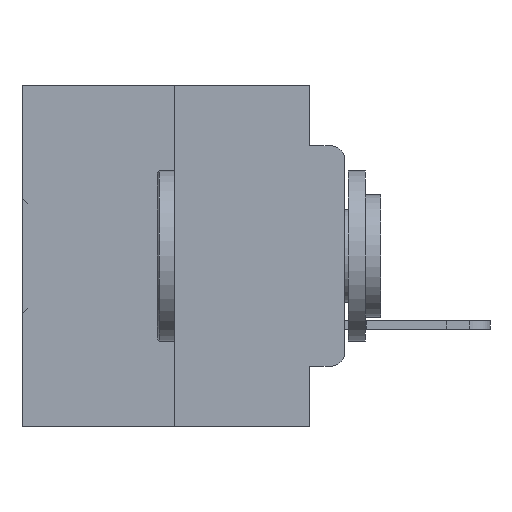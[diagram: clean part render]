
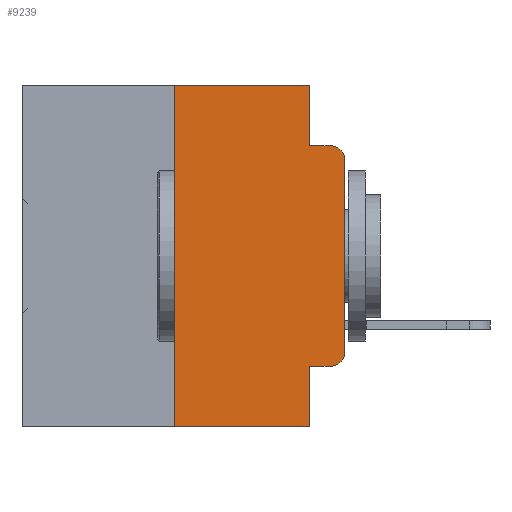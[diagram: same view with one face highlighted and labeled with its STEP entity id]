
A CAD part, left-side view. The second image highlights one B-rep face of the part: STEP entity #9239.
In plain terms, the highlighted planar face has unit normal (-1, 0, 0).
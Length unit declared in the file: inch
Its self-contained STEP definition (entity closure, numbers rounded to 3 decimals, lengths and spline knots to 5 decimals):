
#179 = VECTOR ( 'NONE', #11334, 39.37008 ) ;
#973 = FACE_OUTER_BOUND ( 'NONE', #3663, .T. ) ;
#1327 = CARTESIAN_POINT ( 'NONE',  ( 0., 0.051, -0.0885 ) ) ;
#1749 = CARTESIAN_POINT ( 'NONE',  ( 0., 0.473, 0. ) ) ;
#1759 = DIRECTION ( 'NONE',  ( 0., -1., 0. ) ) ;
#1784 = ORIENTED_EDGE ( 'NONE', *, *, #26303, .T. ) ;
#2339 = DIRECTION ( 'NONE',  ( 0., -1., 0. ) ) ;
#2803 = LINE ( 'NONE', #24411, #24666 ) ;
#3485 = CARTESIAN_POINT ( 'NONE',  ( 0., 0.473, -0.5 ) ) ;
#3663 = EDGE_LOOP ( 'NONE', ( #1784, #11729, #7660, #13972, #16989, #17748, #12508, #15870, #22640, #26390 ) ) ;
#3747 = VERTEX_POINT ( 'NONE', #17767 ) ;
#4022 = VERTEX_POINT ( 'NONE', #1327 ) ;
#4201 = VECTOR ( 'NONE', #25936, 39.37008 ) ;
#5179 = LINE ( 'NONE', #28516, #4201 ) ;
#5334 = CARTESIAN_POINT ( 'NONE',  ( 0., 0.051, -0.0885 ) ) ;
#5476 = VERTEX_POINT ( 'NONE', #19893 ) ;
#5604 = EDGE_CURVE ( 'NONE', #11550, #19818, #31973, .T. ) ;
#5982 = CARTESIAN_POINT ( 'NONE',  ( 0., 0.051, 0. ) ) ;
#6362 = LINE ( 'NONE', #28811, #13258 ) ;
#6499 = DIRECTION ( 'NONE',  ( 0., 0., -1. ) ) ;
#7012 = VERTEX_POINT ( 'NONE', #10464 ) ;
#7660 = ORIENTED_EDGE ( 'NONE', *, *, #20836, .F. ) ;
#8556 = PLANE ( 'NONE',  #15994 ) ;
#8940 = DIRECTION ( 'NONE',  ( 0., 0., 1. ) ) ;
#9149 = CARTESIAN_POINT ( 'NONE',  ( 0., 0.25, 0. ) ) ;
#9239 = ADVANCED_FACE ( 'NONE', ( #973 ), #8556, .F. ) ;
#10116 = EDGE_CURVE ( 'NONE', #14273, #35083, #30186, .T. ) ;
#10464 = CARTESIAN_POINT ( 'NONE',  ( 0., 0.02, -0.0885 ) ) ;
#11184 = LINE ( 'NONE', #5982, #18620 ) ;
#11334 = DIRECTION ( 'NONE',  ( 0., -1., 0. ) ) ;
#11550 = VERTEX_POINT ( 'NONE', #31933 ) ;
#11585 = EDGE_CURVE ( 'NONE', #20948, #11550, #6362, .T. ) ;
#11639 = CARTESIAN_POINT ( 'NONE',  ( 0., 0.25, -0.5 ) ) ;
#11729 = ORIENTED_EDGE ( 'NONE', *, *, #22694, .T. ) ;
#12382 = AXIS2_PLACEMENT_3D ( 'NONE', #14731, #14684, #14679 ) ;
#12508 = ORIENTED_EDGE ( 'NONE', *, *, #10116, .T. ) ;
#12522 = DIRECTION ( 'NONE',  ( 0., 0., -1. ) ) ;
#13258 = VECTOR ( 'NONE', #28668, 39.37008 ) ;
#13535 = EDGE_CURVE ( 'NONE', #20948, #35083, #2803, .T. ) ;
#13877 = DIRECTION ( 'NONE',  ( -1., 0., 0. ) ) ;
#13972 = ORIENTED_EDGE ( 'NONE', *, *, #19061, .F. ) ;
#14273 = VERTEX_POINT ( 'NONE', #11639 ) ;
#14632 = CARTESIAN_POINT ( 'NONE',  ( 0., 0., -0.3915 ) ) ;
#14679 = DIRECTION ( 'NONE',  ( 0., 0., -1. ) ) ;
#14684 = DIRECTION ( 'NONE',  ( -1., 0., 0. ) ) ;
#14731 = CARTESIAN_POINT ( 'NONE',  ( 0., 0.02, -0.3915 ) ) ;
#15371 = EDGE_CURVE ( 'NONE', #14273, #24079, #25806, .T. ) ;
#15619 = EDGE_CURVE ( 'NONE', #24079, #5476, #16378, .T. ) ;
#15870 = ORIENTED_EDGE ( 'NONE', *, *, #13535, .F. ) ;
#15994 = AXIS2_PLACEMENT_3D ( 'NONE', #35100, #34679, #12522 ) ;
#16378 = LINE ( 'NONE', #1749, #29738 ) ;
#16989 = ORIENTED_EDGE ( 'NONE', *, *, #15619, .F. ) ;
#17237 = AXIS2_PLACEMENT_3D ( 'NONE', #29869, #13877, #32298 ) ;
#17571 = CARTESIAN_POINT ( 'NONE',  ( 0., 0.051, -0.4115 ) ) ;
#17748 = ORIENTED_EDGE ( 'NONE', *, *, #15371, .F. ) ;
#17767 = CARTESIAN_POINT ( 'NONE',  ( 0., 0., -0.1085 ) ) ;
#18567 = VECTOR ( 'NONE', #8940, 39.37008 ) ;
#18620 = VECTOR ( 'NONE', #6499, 39.37008 ) ;
#19061 = EDGE_CURVE ( 'NONE', #5476, #4022, #11184, .T. ) ;
#19818 = VERTEX_POINT ( 'NONE', #14632 ) ;
#19893 = CARTESIAN_POINT ( 'NONE',  ( 0., 0.051, 0. ) ) ;
#20836 = EDGE_CURVE ( 'NONE', #4022, #7012, #23173, .T. ) ;
#20948 = VERTEX_POINT ( 'NONE', #17571 ) ;
#21524 = CARTESIAN_POINT ( 'NONE',  ( 0., 0.25, 0. ) ) ;
#22640 = ORIENTED_EDGE ( 'NONE', *, *, #11585, .T. ) ;
#22694 = EDGE_CURVE ( 'NONE', #3747, #7012, #33065, .T. ) ;
#23173 = LINE ( 'NONE', #5334, #179 ) ;
#23341 = VECTOR ( 'NONE', #2339, 39.37008 ) ;
#24079 = VERTEX_POINT ( 'NONE', #21524 ) ;
#24136 = DIRECTION ( 'NONE',  ( 0., 0., -1. ) ) ;
#24411 = CARTESIAN_POINT ( 'NONE',  ( 0., 0.051, 0. ) ) ;
#24666 = VECTOR ( 'NONE', #24136, 39.37008 ) ;
#25806 = LINE ( 'NONE', #9149, #18567 ) ;
#25936 = DIRECTION ( 'NONE',  ( 0., 0., 1. ) ) ;
#26303 = EDGE_CURVE ( 'NONE', #19818, #3747, #5179, .T. ) ;
#26390 = ORIENTED_EDGE ( 'NONE', *, *, #5604, .T. ) ;
#28516 = CARTESIAN_POINT ( 'NONE',  ( 0., 0., 0. ) ) ;
#28668 = DIRECTION ( 'NONE',  ( 0., -1., 0. ) ) ;
#28811 = CARTESIAN_POINT ( 'NONE',  ( 0., 0.051, -0.4115 ) ) ;
#29738 = VECTOR ( 'NONE', #1759, 39.37008 ) ;
#29869 = CARTESIAN_POINT ( 'NONE',  ( 0., 0.02, -0.1085 ) ) ;
#30186 = LINE ( 'NONE', #3485, #23341 ) ;
#30302 = CARTESIAN_POINT ( 'NONE',  ( 0., 0.051, -0.5 ) ) ;
#31933 = CARTESIAN_POINT ( 'NONE',  ( 0., 0.02, -0.4115 ) ) ;
#31973 = CIRCLE ( 'NONE', #12382, 0.02 ) ;
#32298 = DIRECTION ( 'NONE',  ( 0., 0., -1. ) ) ;
#33065 = CIRCLE ( 'NONE', #17237, 0.02 ) ;
#34679 = DIRECTION ( 'NONE',  ( 1., 0., 0. ) ) ;
#35083 = VERTEX_POINT ( 'NONE', #30302 ) ;
#35100 = CARTESIAN_POINT ( 'NONE',  ( 0., 0.473, 0. ) ) ;
